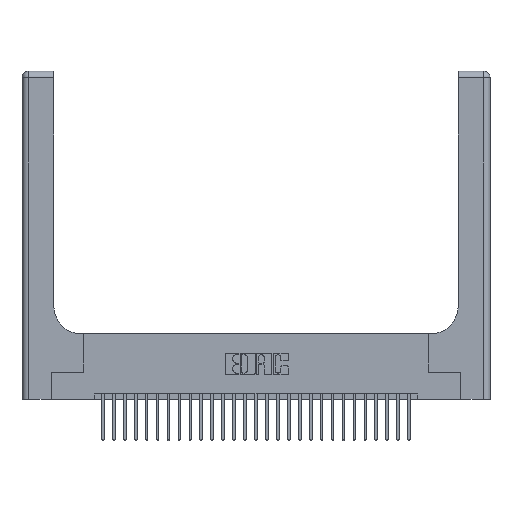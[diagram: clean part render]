
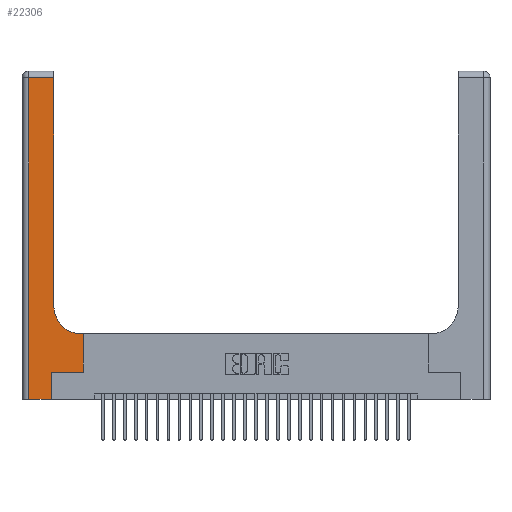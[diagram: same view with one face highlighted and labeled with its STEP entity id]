
A CAD part, top view. The second image highlights one B-rep face of the part: STEP entity #22306.
In plain terms, the highlighted planar face has unit normal (0, 0, 1).
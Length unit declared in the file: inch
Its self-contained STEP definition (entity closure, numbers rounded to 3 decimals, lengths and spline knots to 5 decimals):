
#73 = LINE ( 'NONE', #5051, #2899 ) ;
#621 = VERTEX_POINT ( 'NONE', #18628 ) ;
#693 = LINE ( 'NONE', #27443, #25771 ) ;
#967 = LINE ( 'NONE', #3828, #1238 ) ;
#1194 = AXIS2_PLACEMENT_3D ( 'NONE', #2406, #18431, #18619 ) ;
#1238 = VECTOR ( 'NONE', #15453, 39.37008 ) ;
#1814 = ORIENTED_EDGE ( 'NONE', *, *, #21281, .T. ) ;
#2406 = CARTESIAN_POINT ( 'NONE',  ( 0.5415, 0.85, 0.37 ) ) ;
#2899 = VECTOR ( 'NONE', #21140, 39.37008 ) ;
#2937 = ORIENTED_EDGE ( 'NONE', *, *, #23497, .T. ) ;
#3777 = LINE ( 'NONE', #13453, #12426 ) ;
#3828 = CARTESIAN_POINT ( 'NONE',  ( 0.2915, 0.6, 0.37 ) ) ;
#4437 = LINE ( 'NONE', #21368, #20184 ) ;
#4507 = CARTESIAN_POINT ( 'NONE',  ( 0.5415, 0.6, 0.37 ) ) ;
#5051 = CARTESIAN_POINT ( 'NONE',  ( 0., 0., 0.37 ) ) ;
#5525 = CARTESIAN_POINT ( 'NONE',  ( 0.06, 0., 0.37 ) ) ;
#5622 = VERTEX_POINT ( 'NONE', #5525 ) ;
#6275 = CARTESIAN_POINT ( 'NONE',  ( 0.2915, 3., 0.37 ) ) ;
#6656 = VECTOR ( 'NONE', #29241, 39.37008 ) ;
#6779 = VERTEX_POINT ( 'NONE', #9651 ) ;
#6975 = VERTEX_POINT ( 'NONE', #21443 ) ;
#7361 = CARTESIAN_POINT ( 'NONE',  ( 0.06, 3., 0.37 ) ) ;
#9235 = VERTEX_POINT ( 'NONE', #17892 ) ;
#9489 = DIRECTION ( 'NONE',  ( 1., 0., 0. ) ) ;
#9651 = CARTESIAN_POINT ( 'NONE',  ( 0.269, 0.25, 0.37 ) ) ;
#9746 = ORIENTED_EDGE ( 'NONE', *, *, #25279, .T. ) ;
#9852 = EDGE_CURVE ( 'NONE', #24921, #17139, #19137, .T. ) ;
#9934 = ORIENTED_EDGE ( 'NONE', *, *, #12162, .T. ) ;
#10259 = CARTESIAN_POINT ( 'NONE',  ( 0.5585, 0.25, 0.37 ) ) ;
#10376 = EDGE_LOOP ( 'NONE', ( #23260, #1814, #19001, #2937, #9746, #20416, #20776, #11360, #9934 ) ) ;
#10822 = AXIS2_PLACEMENT_3D ( 'NONE', #20248, #17562, #22196 ) ;
#11360 = ORIENTED_EDGE ( 'NONE', *, *, #11861, .T. ) ;
#11522 = VECTOR ( 'NONE', #9489, 39.37008 ) ;
#11611 = VERTEX_POINT ( 'NONE', #10259 ) ;
#11861 = EDGE_CURVE ( 'NONE', #9235, #24565, #967, .T. ) ;
#12162 = EDGE_CURVE ( 'NONE', #24565, #24921, #25855, .T. ) ;
#12426 = VECTOR ( 'NONE', #15935, 39.37008 ) ;
#12817 = EDGE_CURVE ( 'NONE', #6779, #11611, #21500, .T. ) ;
#13453 = CARTESIAN_POINT ( 'NONE',  ( 0., 2.94, 0.37 ) ) ;
#13515 = LINE ( 'NONE', #7361, #18136 ) ;
#13616 = CARTESIAN_POINT ( 'NONE',  ( 0.269, 0.25, 0.37 ) ) ;
#14125 = FACE_OUTER_BOUND ( 'NONE', #10376, .T. ) ;
#14977 = PLANE ( 'NONE',  #10822 ) ;
#15002 = EDGE_CURVE ( 'NONE', #621, #5622, #13515, .T. ) ;
#15453 = DIRECTION ( 'NONE',  ( -1., 0., 0. ) ) ;
#15935 = DIRECTION ( 'NONE',  ( -1., 0., 0. ) ) ;
#17139 = VERTEX_POINT ( 'NONE', #26758 ) ;
#17287 = EDGE_CURVE ( 'NONE', #11611, #9235, #4437, .T. ) ;
#17562 = DIRECTION ( 'NONE',  ( 0., 0., -1. ) ) ;
#17892 = CARTESIAN_POINT ( 'NONE',  ( 0.5585, 0.6, 0.37 ) ) ;
#18136 = VECTOR ( 'NONE', #20843, 39.37008 ) ;
#18431 = DIRECTION ( 'NONE',  ( 0., 0., -1. ) ) ;
#18619 = DIRECTION ( 'NONE',  ( 1., 0., 0. ) ) ;
#18628 = CARTESIAN_POINT ( 'NONE',  ( 0.06, 2.94, 0.37 ) ) ;
#18954 = DIRECTION ( 'NONE',  ( 0., 1., 0. ) ) ;
#19001 = ORIENTED_EDGE ( 'NONE', *, *, #15002, .T. ) ;
#19137 = LINE ( 'NONE', #6275, #6656 ) ;
#20184 = VECTOR ( 'NONE', #18954, 39.37008 ) ;
#20248 = CARTESIAN_POINT ( 'NONE',  ( 0., 3., 0.37 ) ) ;
#20416 = ORIENTED_EDGE ( 'NONE', *, *, #12817, .T. ) ;
#20776 = ORIENTED_EDGE ( 'NONE', *, *, #17287, .T. ) ;
#20843 = DIRECTION ( 'NONE',  ( 0., -1., 0. ) ) ;
#21140 = DIRECTION ( 'NONE',  ( 1., 0., 0. ) ) ;
#21281 = EDGE_CURVE ( 'NONE', #17139, #621, #3777, .T. ) ;
#21368 = CARTESIAN_POINT ( 'NONE',  ( 0.5585, 0.25, 0.37 ) ) ;
#21443 = CARTESIAN_POINT ( 'NONE',  ( 0.269, 0., 0.37 ) ) ;
#21500 = LINE ( 'NONE', #13616, #11522 ) ;
#21706 = CARTESIAN_POINT ( 'NONE',  ( 0.2915, 0.85, 0.37 ) ) ;
#22196 = DIRECTION ( 'NONE',  ( -1., 0., 0. ) ) ;
#22306 = ADVANCED_FACE ( 'NONE', ( #14125 ), #14977, .F. ) ;
#23260 = ORIENTED_EDGE ( 'NONE', *, *, #9852, .T. ) ;
#23384 = DIRECTION ( 'NONE',  ( 0., 1., 0. ) ) ;
#23497 = EDGE_CURVE ( 'NONE', #5622, #6975, #73, .T. ) ;
#24565 = VERTEX_POINT ( 'NONE', #4507 ) ;
#24921 = VERTEX_POINT ( 'NONE', #21706 ) ;
#25279 = EDGE_CURVE ( 'NONE', #6975, #6779, #693, .T. ) ;
#25771 = VECTOR ( 'NONE', #23384, 39.37008 ) ;
#25855 = CIRCLE ( 'NONE', #1194, 0.25 ) ;
#26758 = CARTESIAN_POINT ( 'NONE',  ( 0.2915, 2.94, 0.37 ) ) ;
#27443 = CARTESIAN_POINT ( 'NONE',  ( 0.269, 0., 0.37 ) ) ;
#29241 = DIRECTION ( 'NONE',  ( 0., 1., 0. ) ) ;
